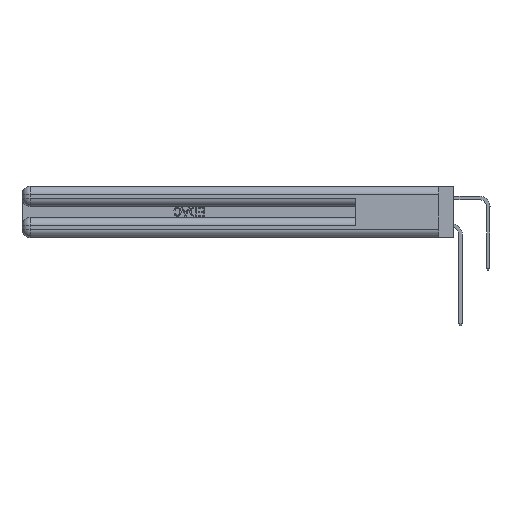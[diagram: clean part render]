
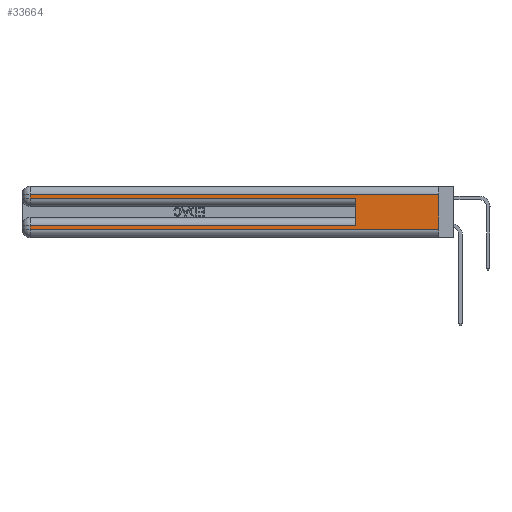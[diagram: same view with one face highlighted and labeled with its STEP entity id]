
A CAD part, left-side view. The second image highlights one B-rep face of the part: STEP entity #33664.
In plain terms, the highlighted planar face has unit normal (-1, 0, 0).
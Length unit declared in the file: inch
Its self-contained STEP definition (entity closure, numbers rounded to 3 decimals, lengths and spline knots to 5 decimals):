
#991 = VERTEX_POINT ( 'NONE', #35799 ) ;
#1260 = DIRECTION ( 'NONE',  ( 1., 0., 0. ) ) ;
#2208 = VECTOR ( 'NONE', #4586, 39.37008 ) ;
#3098 = DIRECTION ( 'NONE',  ( 0., 1., 0. ) ) ;
#3547 = CARTESIAN_POINT ( 'NONE',  ( 0., 2.94, 0.06 ) ) ;
#4568 = EDGE_CURVE ( 'NONE', #991, #19732, #7864, .T. ) ;
#4586 = DIRECTION ( 'NONE',  ( 0., 0., -1. ) ) ;
#6773 = DIRECTION ( 'NONE',  ( 0., 0., -1. ) ) ;
#7028 = CARTESIAN_POINT ( 'NONE',  ( 0., 0., 0.31 ) ) ;
#7659 = VECTOR ( 'NONE', #34247, 39.37008 ) ;
#7864 = LINE ( 'NONE', #19058, #29496 ) ;
#8390 = VERTEX_POINT ( 'NONE', #18957 ) ;
#10177 = ORIENTED_EDGE ( 'NONE', *, *, #31722, .T. ) ;
#11996 = VERTEX_POINT ( 'NONE', #23525 ) ;
#13987 = LINE ( 'NONE', #41233, #16565 ) ;
#14309 = CARTESIAN_POINT ( 'NONE',  ( 0., 0., 0.37 ) ) ;
#14625 = LINE ( 'NONE', #35244, #33651 ) ;
#15540 = AXIS2_PLACEMENT_3D ( 'NONE', #14309, #1260, #17464 ) ;
#15692 = DIRECTION ( 'NONE',  ( 0., -1., 0. ) ) ;
#16121 = CARTESIAN_POINT ( 'NONE',  ( 0., 0., 0.085 ) ) ;
#16565 = VECTOR ( 'NONE', #35935, 39.37008 ) ;
#16611 = FACE_OUTER_BOUND ( 'NONE', #35764, .T. ) ;
#16828 = ORIENTED_EDGE ( 'NONE', *, *, #27640, .T. ) ;
#17464 = DIRECTION ( 'NONE',  ( 0., 0., -1. ) ) ;
#18354 = VERTEX_POINT ( 'NONE', #38768 ) ;
#18957 = CARTESIAN_POINT ( 'NONE',  ( 0., 0.6, 0.085 ) ) ;
#19058 = CARTESIAN_POINT ( 'NONE',  ( 0., 2.94, 0.37 ) ) ;
#19732 = VERTEX_POINT ( 'NONE', #3547 ) ;
#20080 = ORIENTED_EDGE ( 'NONE', *, *, #40973, .F. ) ;
#21214 = VECTOR ( 'NONE', #6773, 39.37008 ) ;
#22771 = LINE ( 'NONE', #34180, #2208 ) ;
#23381 = CARTESIAN_POINT ( 'NONE',  ( 0., 2.94, 0.285 ) ) ;
#23525 = CARTESIAN_POINT ( 'NONE',  ( 0., 0., 0.06 ) ) ;
#25074 = LINE ( 'NONE', #36918, #30711 ) ;
#25160 = LINE ( 'NONE', #30637, #7659 ) ;
#26078 = ORIENTED_EDGE ( 'NONE', *, *, #29250, .F. ) ;
#26204 = EDGE_CURVE ( 'NONE', #36632, #38271, #35149, .T. ) ;
#26589 = EDGE_CURVE ( 'NONE', #29773, #36632, #13987, .T. ) ;
#27640 = EDGE_CURVE ( 'NONE', #8390, #991, #36624, .T. ) ;
#28654 = ORIENTED_EDGE ( 'NONE', *, *, #30169, .T. ) ;
#29250 = EDGE_CURVE ( 'NONE', #8390, #18354, #25160, .T. ) ;
#29273 = CARTESIAN_POINT ( 'NONE',  ( 0., 2.94, 0.37 ) ) ;
#29422 = VECTOR ( 'NONE', #3098, 39.37008 ) ;
#29496 = VECTOR ( 'NONE', #38661, 39.37008 ) ;
#29773 = VERTEX_POINT ( 'NONE', #7028 ) ;
#30169 = EDGE_CURVE ( 'NONE', #38271, #18354, #25074, .T. ) ;
#30637 = CARTESIAN_POINT ( 'NONE',  ( 0., 0.6, 0.145 ) ) ;
#30711 = VECTOR ( 'NONE', #34189, 39.37008 ) ;
#31722 = EDGE_CURVE ( 'NONE', #19732, #11996, #14625, .T. ) ;
#32398 = CARTESIAN_POINT ( 'NONE',  ( 0., 2.94, 0.31 ) ) ;
#33651 = VECTOR ( 'NONE', #15692, 39.37008 ) ;
#33664 = ADVANCED_FACE ( 'NONE', ( #16611 ), #40635, .F. ) ;
#33829 = ORIENTED_EDGE ( 'NONE', *, *, #26204, .T. ) ;
#34180 = CARTESIAN_POINT ( 'NONE',  ( 0., 0., 0.37 ) ) ;
#34189 = DIRECTION ( 'NONE',  ( 0., -1., 0. ) ) ;
#34247 = DIRECTION ( 'NONE',  ( 0., 0., 1. ) ) ;
#35149 = LINE ( 'NONE', #29273, #21214 ) ;
#35244 = CARTESIAN_POINT ( 'NONE',  ( 0., 0., 0.06 ) ) ;
#35764 = EDGE_LOOP ( 'NONE', ( #20080, #42455, #33829, #28654, #26078, #16828, #35780, #10177 ) ) ;
#35780 = ORIENTED_EDGE ( 'NONE', *, *, #4568, .T. ) ;
#35799 = CARTESIAN_POINT ( 'NONE',  ( 0., 2.94, 0.085 ) ) ;
#35935 = DIRECTION ( 'NONE',  ( 0., 1., 0. ) ) ;
#36624 = LINE ( 'NONE', #16121, #29422 ) ;
#36632 = VERTEX_POINT ( 'NONE', #32398 ) ;
#36918 = CARTESIAN_POINT ( 'NONE',  ( 0., 0., 0.285 ) ) ;
#38271 = VERTEX_POINT ( 'NONE', #23381 ) ;
#38661 = DIRECTION ( 'NONE',  ( 0., 0., -1. ) ) ;
#38768 = CARTESIAN_POINT ( 'NONE',  ( 0., 0.6, 0.285 ) ) ;
#40635 = PLANE ( 'NONE',  #15540 ) ;
#40973 = EDGE_CURVE ( 'NONE', #29773, #11996, #22771, .T. ) ;
#41233 = CARTESIAN_POINT ( 'NONE',  ( 0., 0., 0.31 ) ) ;
#42455 = ORIENTED_EDGE ( 'NONE', *, *, #26589, .T. ) ;
